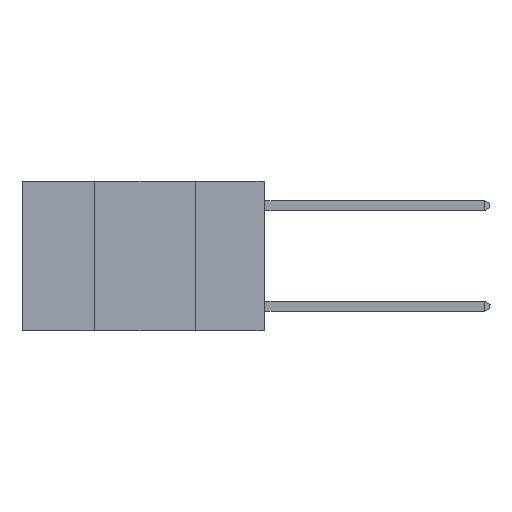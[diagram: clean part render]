
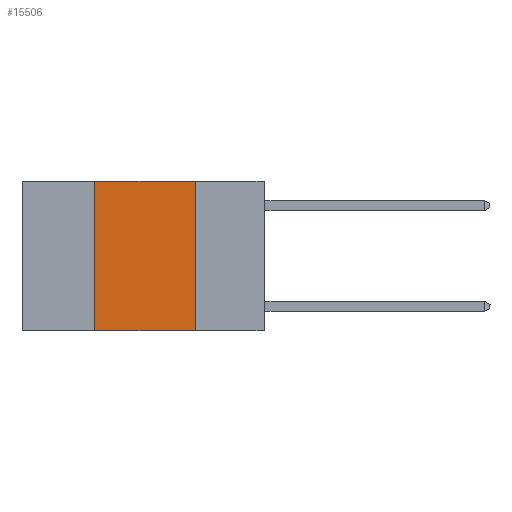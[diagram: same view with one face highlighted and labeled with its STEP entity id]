
A CAD part, left-side view. The second image highlights one B-rep face of the part: STEP entity #15506.
In plain terms, the highlighted planar face has unit normal (-1, 0, 0).
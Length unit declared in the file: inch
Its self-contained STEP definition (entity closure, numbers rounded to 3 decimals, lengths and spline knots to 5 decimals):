
#459 = DIRECTION ( 'NONE',  ( 1., 0., 0. ) ) ;
#2157 = EDGE_CURVE ( 'NONE', #4812, #15834, #3484, .T. ) ;
#3484 = LINE ( 'NONE', #8509, #21675 ) ;
#4812 = VERTEX_POINT ( 'NONE', #11672 ) ;
#4967 = VECTOR ( 'NONE', #22153, 39.37008 ) ;
#5023 = CARTESIAN_POINT ( 'NONE',  ( 0., 0.42, 0. ) ) ;
#5824 = ORIENTED_EDGE ( 'NONE', *, *, #2157, .F. ) ;
#5857 = VECTOR ( 'NONE', #22029, 39.37008 ) ;
#6829 = EDGE_LOOP ( 'NONE', ( #22265, #14179, #5824, #15844 ) ) ;
#8087 = VERTEX_POINT ( 'NONE', #13019 ) ;
#8265 = EDGE_CURVE ( 'NONE', #4812, #8087, #18528, .T. ) ;
#8509 = CARTESIAN_POINT ( 'NONE',  ( 0., 0.42, 0. ) ) ;
#9981 = CARTESIAN_POINT ( 'NONE',  ( 0., 0.6, -0.37 ) ) ;
#11672 = CARTESIAN_POINT ( 'NONE',  ( 0., 0.42, -0.37 ) ) ;
#12068 = DIRECTION ( 'NONE',  ( 0., 0., 1. ) ) ;
#13019 = CARTESIAN_POINT ( 'NONE',  ( 0., 0.17, -0.37 ) ) ;
#13076 = DIRECTION ( 'NONE',  ( 0., 0., -1. ) ) ;
#13275 = CARTESIAN_POINT ( 'NONE',  ( 0., 0.17, 0. ) ) ;
#14179 = ORIENTED_EDGE ( 'NONE', *, *, #19314, .F. ) ;
#14217 = VERTEX_POINT ( 'NONE', #13275 ) ;
#14432 = FACE_OUTER_BOUND ( 'NONE', #6829, .T. ) ;
#14737 = VECTOR ( 'NONE', #18918, 39.37008 ) ;
#15287 = LINE ( 'NONE', #17198, #14737 ) ;
#15506 = ADVANCED_FACE ( 'NONE', ( #14432 ), #19990, .F. ) ;
#15834 = VERTEX_POINT ( 'NONE', #5023 ) ;
#15844 = ORIENTED_EDGE ( 'NONE', *, *, #8265, .T. ) ;
#16864 = CARTESIAN_POINT ( 'NONE',  ( 0., 0.6, 0. ) ) ;
#17198 = CARTESIAN_POINT ( 'NONE',  ( 0., 0.17, 0. ) ) ;
#18528 = LINE ( 'NONE', #9981, #4967 ) ;
#18918 = DIRECTION ( 'NONE',  ( 0., 0., -1. ) ) ;
#19314 = EDGE_CURVE ( 'NONE', #15834, #14217, #19911, .T. ) ;
#19911 = LINE ( 'NONE', #16864, #5857 ) ;
#19990 = PLANE ( 'NONE',  #22521 ) ;
#20427 = EDGE_CURVE ( 'NONE', #14217, #8087, #15287, .T. ) ;
#21675 = VECTOR ( 'NONE', #12068, 39.37008 ) ;
#21701 = CARTESIAN_POINT ( 'NONE',  ( 0., 0.6, 0. ) ) ;
#22029 = DIRECTION ( 'NONE',  ( 0., -1., 0. ) ) ;
#22153 = DIRECTION ( 'NONE',  ( 0., -1., 0. ) ) ;
#22265 = ORIENTED_EDGE ( 'NONE', *, *, #20427, .F. ) ;
#22521 = AXIS2_PLACEMENT_3D ( 'NONE', #21701, #459, #13076 ) ;
